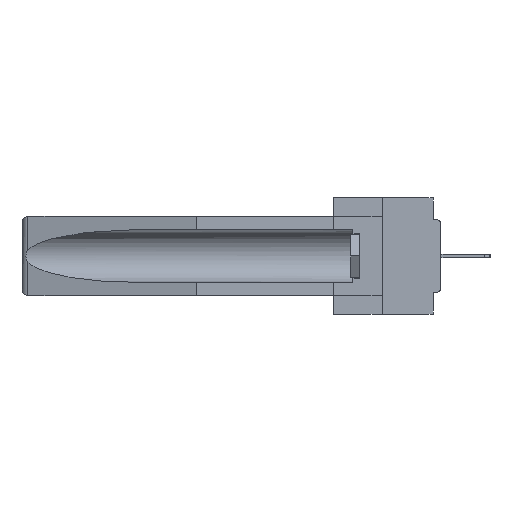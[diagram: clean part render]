
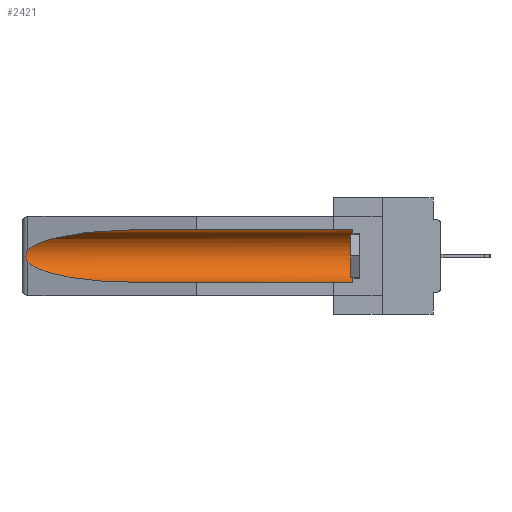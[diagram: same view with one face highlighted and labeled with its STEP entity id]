
A CAD part, left-side view. The second image highlights one B-rep face of the part: STEP entity #2421.
In plain terms, the highlighted cylindrical face has radius 2.857 mm (diameter 5.715 mm), a partial arc.
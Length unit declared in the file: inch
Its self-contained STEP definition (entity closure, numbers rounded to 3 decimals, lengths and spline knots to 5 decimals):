
#736 = CARTESIAN_POINT ( 'NONE',  ( 0.155, 1.07973, -0.059 ) ) ;
#979 = CARTESIAN_POINT ( 'NONE',  ( 0.26537, 1.52718, -0.14972 ) ) ;
#1085 = CARTESIAN_POINT ( 'NONE',  ( 0.26597, 1.5296, -0.19026 ) ) ;
#1279 = VECTOR ( 'NONE', #21345, 39.37008 ) ;
#1636 = ORIENTED_EDGE ( 'NONE', *, *, #28508, .T. ) ;
#2421 = ADVANCED_FACE ( 'NONE', ( #22710 ), #8944, .F. ) ;
#2961 = ORIENTED_EDGE ( 'NONE', *, *, #8401, .F. ) ;
#3609 = CARTESIAN_POINT ( 'NONE',  ( 0.26597, 1.52961, -0.15275 ) ) ;
#3986 = CARTESIAN_POINT ( 'NONE',  ( 0.25451, 1.48313, -0.24835 ) ) ;
#4004 = DIRECTION ( 'NONE',  ( 0., 0., 1. ) ) ;
#4059 = CARTESIAN_POINT ( 'NONE',  ( 0.26537, 1.52718, -0.14972 ) ) ;
#4776 = CARTESIAN_POINT ( 'NONE',  ( 0.155, 0.126, -0.284 ) ) ;
#4793 = AXIS2_PLACEMENT_3D ( 'NONE', #25225, #9728, #27777 ) ;
#4898 = CARTESIAN_POINT ( 'NONE',  ( 0.155, 1.07973, -0.059 ) ) ;
#5046 = AXIS2_PLACEMENT_3D ( 'NONE', #10281, #5585, #4004 ) ;
#5585 = DIRECTION ( 'NONE',  ( 0., 1., 0. ) ) ;
#7955 = CARTESIAN_POINT ( 'NONE',  ( 0.155, 1.07973, -0.284 ) ) ;
#8238 = ORIENTED_EDGE ( 'NONE', *, *, #15361, .T. ) ;
#8401 = EDGE_CURVE ( 'NONE', #12218, #26132, #28831, .T. ) ;
#8476 = CIRCLE ( 'NONE', #4793, 0.1125 ) ;
#8944 = CYLINDRICAL_SURFACE ( 'NONE', #5046, 0.1125 ) ;
#9143 = VERTEX_POINT ( 'NONE', #32399 ) ;
#9223 = CARTESIAN_POINT ( 'NONE',  ( 0.155, 1.07973, -0.284 ) ) ;
#9728 = DIRECTION ( 'NONE',  ( 0., -1., 0. ) ) ;
#10139 = CARTESIAN_POINT ( 'NONE',  ( 0.25451, 1.48313, -0.09465 ) ) ;
#10281 = CARTESIAN_POINT ( 'NONE',  ( 0.155, -0.30754, -0.1715 ) ) ;
#10339 =( BOUNDED_CURVE ( )  B_SPLINE_CURVE ( 3, ( #22119, #3986, #24730, #9223 ),
 .UNSPECIFIED., .F., .F. ) 
 B_SPLINE_CURVE_WITH_KNOTS ( ( 4, 4 ),
 ( 0.1948, 1.5708 ),
 .UNSPECIFIED. ) 
 CURVE ( )  GEOMETRIC_REPRESENTATION_ITEM ( )  RATIONAL_B_SPLINE_CURVE ( ( 1., 0.848, 0.848, 1. ) ) 
 REPRESENTATION_ITEM ( '' )  );
#10561 =( BOUNDED_CURVE ( )  B_SPLINE_CURVE ( 3, ( #4898, #20447, #10139, #28175 ),
 .UNSPECIFIED., .F., .F. ) 
 B_SPLINE_CURVE_WITH_KNOTS ( ( 4, 4 ),
 ( 4.71239, 6.08839 ),
 .UNSPECIFIED. ) 
 CURVE ( )  GEOMETRIC_REPRESENTATION_ITEM ( )  RATIONAL_B_SPLINE_CURVE ( ( 1., 0.848, 0.848, 1. ) ) 
 REPRESENTATION_ITEM ( '' )  );
#10884 = B_SPLINE_CURVE_WITH_KNOTS ( 'NONE', 3,
 ( #979, #3609, #26938, #11491, #29505, #14082, #32082, #16709, #1085, #19304 ),
 .UNSPECIFIED., .F., .F.,
 ( 4, 2, 2, 2, 4 ),
 ( 0., 0.00029, 0.00058, 0.00087, 0.00117 ),
 .UNSPECIFIED. ) ;
#11491 = CARTESIAN_POINT ( 'NONE',  ( 0.2673, 1.5327, -0.16383 ) ) ;
#11617 = CARTESIAN_POINT ( 'NONE',  ( 0.155, 0.126, -0.059 ) ) ;
#11659 = ORIENTED_EDGE ( 'NONE', *, *, #31514, .T. ) ;
#12218 = VERTEX_POINT ( 'NONE', #4776 ) ;
#14082 = CARTESIAN_POINT ( 'NONE',  ( 0.2675, 1.53308, -0.17534 ) ) ;
#15361 = EDGE_CURVE ( 'NONE', #21492, #9143, #10884, .T. ) ;
#16160 = CARTESIAN_POINT ( 'NONE',  ( 0.155, -0.30754, -0.284 ) ) ;
#16539 = VECTOR ( 'NONE', #23374, 39.37008 ) ;
#16709 = CARTESIAN_POINT ( 'NONE',  ( 0.26655, 1.53094, -0.18657 ) ) ;
#16885 = LINE ( 'NONE', #20801, #16539 ) ;
#16946 = EDGE_CURVE ( 'NONE', #26261, #21492, #10561, .T. ) ;
#19304 = CARTESIAN_POINT ( 'NONE',  ( 0.26537, 1.52718, -0.19328 ) ) ;
#20447 = CARTESIAN_POINT ( 'NONE',  ( 0.21114, 1.30732, -0.059 ) ) ;
#20569 = EDGE_CURVE ( 'NONE', #12218, #20917, #8476, .T. ) ;
#20801 = CARTESIAN_POINT ( 'NONE',  ( 0.155, -0.30754, -0.059 ) ) ;
#20917 = VERTEX_POINT ( 'NONE', #11617 ) ;
#21345 = DIRECTION ( 'NONE',  ( 0., 1., 0. ) ) ;
#21492 = VERTEX_POINT ( 'NONE', #4059 ) ;
#22119 = CARTESIAN_POINT ( 'NONE',  ( 0.26537, 1.52718, -0.19328 ) ) ;
#22710 = FACE_OUTER_BOUND ( 'NONE', #27921, .T. ) ;
#23374 = DIRECTION ( 'NONE',  ( 0., 1., 0. ) ) ;
#24506 = ORIENTED_EDGE ( 'NONE', *, *, #16946, .T. ) ;
#24730 = CARTESIAN_POINT ( 'NONE',  ( 0.21114, 1.30732, -0.284 ) ) ;
#25225 = CARTESIAN_POINT ( 'NONE',  ( 0.155, 0.126, -0.1715 ) ) ;
#26132 = VERTEX_POINT ( 'NONE', #7955 ) ;
#26261 = VERTEX_POINT ( 'NONE', #736 ) ;
#26938 = CARTESIAN_POINT ( 'NONE',  ( 0.26654, 1.53092, -0.15636 ) ) ;
#27777 = DIRECTION ( 'NONE',  ( 0., 0., 1. ) ) ;
#27921 = EDGE_LOOP ( 'NONE', ( #24506, #8238, #1636, #2961, #28171, #11659 ) ) ;
#28171 = ORIENTED_EDGE ( 'NONE', *, *, #20569, .T. ) ;
#28175 = CARTESIAN_POINT ( 'NONE',  ( 0.26537, 1.52718, -0.14972 ) ) ;
#28508 = EDGE_CURVE ( 'NONE', #9143, #26132, #10339, .T. ) ;
#28831 = LINE ( 'NONE', #16160, #1279 ) ;
#29505 = CARTESIAN_POINT ( 'NONE',  ( 0.2675, 1.53308, -0.16763 ) ) ;
#31514 = EDGE_CURVE ( 'NONE', #20917, #26261, #16885, .T. ) ;
#32082 = CARTESIAN_POINT ( 'NONE',  ( 0.2673, 1.53269, -0.17917 ) ) ;
#32399 = CARTESIAN_POINT ( 'NONE',  ( 0.26537, 1.52718, -0.19328 ) ) ;
